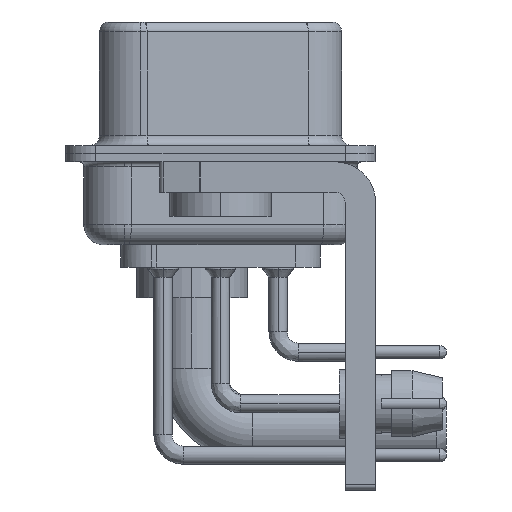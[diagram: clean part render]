
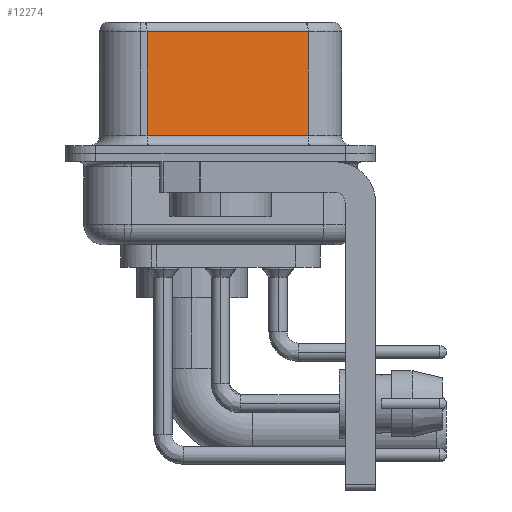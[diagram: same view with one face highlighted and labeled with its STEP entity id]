
A CAD part, left-side view. The second image highlights one B-rep face of the part: STEP entity #12274.
In plain terms, the highlighted planar face has unit normal (-0.985, -0.174, 0).
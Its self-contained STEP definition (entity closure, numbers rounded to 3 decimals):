
#1592 = DIRECTION ( 'NONE',  ( -0.174, 0.985, 0. ) ) ;
#2808 = VECTOR ( 'NONE', #23636, 1000. ) ;
#4668 = VERTEX_POINT ( 'NONE', #16557 ) ;
#8662 = LINE ( 'NONE', #26334, #28873 ) ;
#8815 = DIRECTION ( 'NONE',  ( -0.174, 0.985, 0. ) ) ;
#9785 = EDGE_CURVE ( 'NONE', #10221, #12804, #8662, .T. ) ;
#10221 = VERTEX_POINT ( 'NONE', #26292 ) ;
#10551 = VECTOR ( 'NONE', #8815, 1000. ) ;
#11635 = ORIENTED_EDGE ( 'NONE', *, *, #9785, .F. ) ;
#11641 = LINE ( 'NONE', #20288, #2808 ) ;
#12274 = ADVANCED_FACE ( 'NONE', ( #17296 ), #19661, .F. ) ;
#12657 = VECTOR ( 'NONE', #32289, 1000. ) ;
#12804 = VERTEX_POINT ( 'NONE', #28847 ) ;
#14808 = EDGE_CURVE ( 'NONE', #10221, #31117, #24513, .T. ) ;
#16557 = CARTESIAN_POINT ( 'NONE',  ( 3.73, 3.628, 0.9 ) ) ;
#16740 = ORIENTED_EDGE ( 'NONE', *, *, #22817, .T. ) ;
#16909 = CARTESIAN_POINT ( 'NONE',  ( 5.132, -4.322, 6.52 ) ) ;
#17296 = FACE_OUTER_BOUND ( 'NONE', #34466, .T. ) ;
#17552 = CARTESIAN_POINT ( 'NONE',  ( 5.132, -4.322, 0.9 ) ) ;
#17751 = LINE ( 'NONE', #17552, #12657 ) ;
#18606 = CARTESIAN_POINT ( 'NONE',  ( 5.132, -4.322, 6.02 ) ) ;
#19661 = PLANE ( 'NONE',  #38686 ) ;
#20288 = CARTESIAN_POINT ( 'NONE',  ( 3.73, 3.628, 6.52 ) ) ;
#20408 = ORIENTED_EDGE ( 'NONE', *, *, #35916, .T. ) ;
#22817 = EDGE_CURVE ( 'NONE', #31117, #4668, #11641, .T. ) ;
#23636 = DIRECTION ( 'NONE',  ( 0., 0., -1. ) ) ;
#24513 = LINE ( 'NONE', #18606, #10551 ) ;
#26292 = CARTESIAN_POINT ( 'NONE',  ( 5.132, -4.322, 6.02 ) ) ;
#26334 = CARTESIAN_POINT ( 'NONE',  ( 5.132, -4.322, 6.52 ) ) ;
#28847 = CARTESIAN_POINT ( 'NONE',  ( 5.132, -4.322, 0.9 ) ) ;
#28873 = VECTOR ( 'NONE', #38696, 1000. ) ;
#29283 = DIRECTION ( 'NONE',  ( 0.985, 0.174, 0. ) ) ;
#31117 = VERTEX_POINT ( 'NONE', #37484 ) ;
#31701 = ORIENTED_EDGE ( 'NONE', *, *, #14808, .T. ) ;
#32289 = DIRECTION ( 'NONE',  ( 0.174, -0.985, 0. ) ) ;
#34466 = EDGE_LOOP ( 'NONE', ( #11635, #31701, #16740, #20408 ) ) ;
#35916 = EDGE_CURVE ( 'NONE', #4668, #12804, #17751, .T. ) ;
#37484 = CARTESIAN_POINT ( 'NONE',  ( 3.73, 3.628, 6.02 ) ) ;
#38686 = AXIS2_PLACEMENT_3D ( 'NONE', #16909, #29283, #1592 ) ;
#38696 = DIRECTION ( 'NONE',  ( 0., 0., -1. ) ) ;
